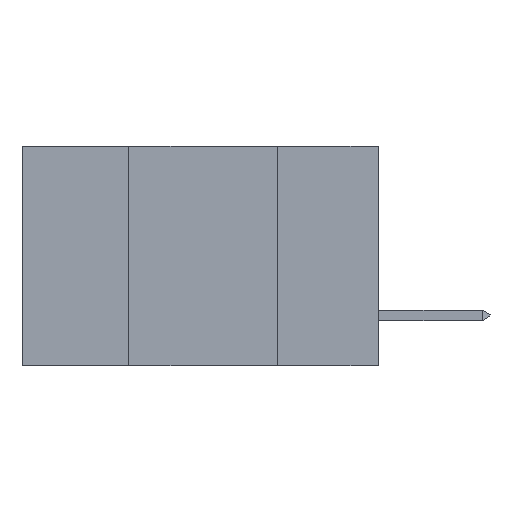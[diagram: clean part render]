
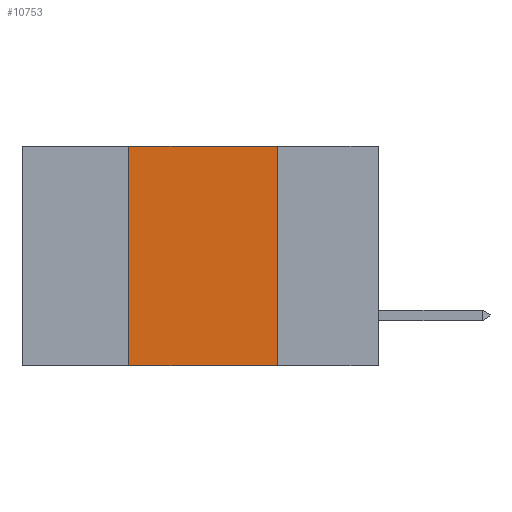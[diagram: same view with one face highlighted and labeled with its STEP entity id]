
A CAD part, left-side view. The second image highlights one B-rep face of the part: STEP entity #10753.
In plain terms, the highlighted planar face has unit normal (-1, 0, 0).
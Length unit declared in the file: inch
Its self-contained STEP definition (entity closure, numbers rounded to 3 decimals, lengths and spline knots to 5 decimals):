
#245 = DIRECTION ( 'NONE',  ( 1., 0., 0. ) ) ;
#306 = VERTEX_POINT ( 'NONE', #3925 ) ;
#405 = VECTOR ( 'NONE', #4376, 39.37008 ) ;
#565 = VECTOR ( 'NONE', #7576, 39.37008 ) ;
#1078 = VERTEX_POINT ( 'NONE', #3845 ) ;
#1709 = EDGE_CURVE ( 'NONE', #6420, #306, #6622, .T. ) ;
#1829 = EDGE_CURVE ( 'NONE', #9556, #306, #8811, .T. ) ;
#2101 = CARTESIAN_POINT ( 'NONE',  ( 0., 0.6, -0.37 ) ) ;
#2388 = CARTESIAN_POINT ( 'NONE',  ( 0., 0.17, -0.37 ) ) ;
#2781 = ORIENTED_EDGE ( 'NONE', *, *, #1709, .T. ) ;
#3845 = CARTESIAN_POINT ( 'NONE',  ( 0., 0.42, 0. ) ) ;
#3925 = CARTESIAN_POINT ( 'NONE',  ( 0., 0.17, -0.37 ) ) ;
#4376 = DIRECTION ( 'NONE',  ( 0., -1., 0. ) ) ;
#4764 = CARTESIAN_POINT ( 'NONE',  ( 0., 0.6, 0. ) ) ;
#4924 = ORIENTED_EDGE ( 'NONE', *, *, #7124, .F. ) ;
#5319 = LINE ( 'NONE', #11452, #405 ) ;
#5908 = DIRECTION ( 'NONE',  ( 0., 0., -1. ) ) ;
#6420 = VERTEX_POINT ( 'NONE', #10943 ) ;
#6599 = LINE ( 'NONE', #7377, #9820 ) ;
#6622 = LINE ( 'NONE', #2101, #565 ) ;
#6708 = ORIENTED_EDGE ( 'NONE', *, *, #1829, .F. ) ;
#6840 = VECTOR ( 'NONE', #10640, 39.37008 ) ;
#7124 = EDGE_CURVE ( 'NONE', #1078, #9556, #5319, .T. ) ;
#7377 = CARTESIAN_POINT ( 'NONE',  ( 0., 0.42, -0.37 ) ) ;
#7576 = DIRECTION ( 'NONE',  ( 0., -1., 0. ) ) ;
#7894 = CARTESIAN_POINT ( 'NONE',  ( 0., 0.17, 0. ) ) ;
#8811 = LINE ( 'NONE', #2388, #6840 ) ;
#9272 = EDGE_LOOP ( 'NONE', ( #6708, #4924, #11270, #2781 ) ) ;
#9331 = DIRECTION ( 'NONE',  ( 0., 0., 1. ) ) ;
#9450 = FACE_OUTER_BOUND ( 'NONE', #9272, .T. ) ;
#9495 = EDGE_CURVE ( 'NONE', #6420, #1078, #6599, .T. ) ;
#9556 = VERTEX_POINT ( 'NONE', #7894 ) ;
#9820 = VECTOR ( 'NONE', #9331, 39.37008 ) ;
#10155 = PLANE ( 'NONE',  #11710 ) ;
#10640 = DIRECTION ( 'NONE',  ( 0., 0., -1. ) ) ;
#10753 = ADVANCED_FACE ( 'NONE', ( #9450 ), #10155, .F. ) ;
#10943 = CARTESIAN_POINT ( 'NONE',  ( 0., 0.42, -0.37 ) ) ;
#11270 = ORIENTED_EDGE ( 'NONE', *, *, #9495, .F. ) ;
#11452 = CARTESIAN_POINT ( 'NONE',  ( 0., 0.6, 0. ) ) ;
#11710 = AXIS2_PLACEMENT_3D ( 'NONE', #4764, #245, #5908 ) ;
